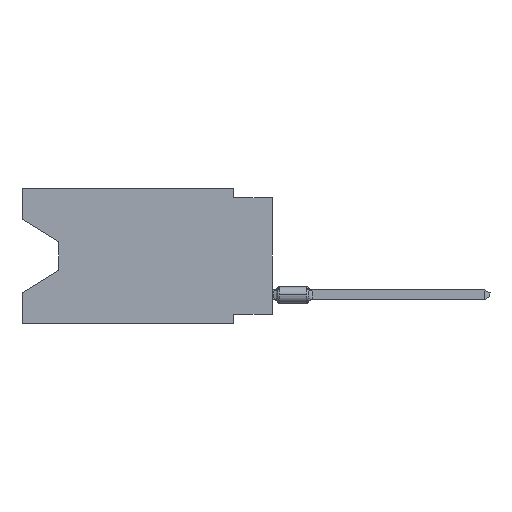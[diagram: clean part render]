
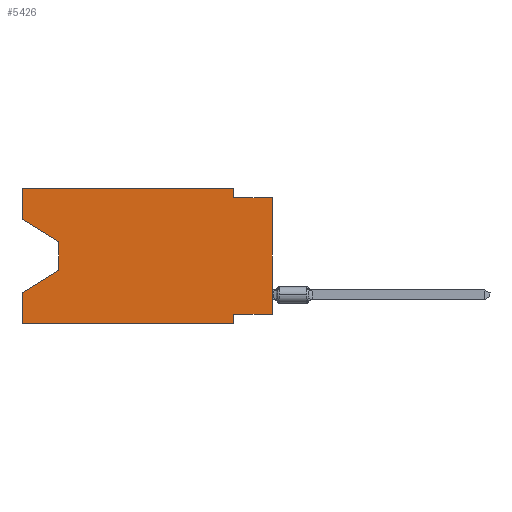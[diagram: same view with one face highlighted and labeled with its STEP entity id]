
A CAD part, left-side view. The second image highlights one B-rep face of the part: STEP entity #5426.
In plain terms, the highlighted planar face has unit normal (-1, 0, 0).
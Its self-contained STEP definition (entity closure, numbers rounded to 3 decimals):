
#700 = CARTESIAN_POINT ( 'NONE',  ( 0., 0., -0.635 ) ) ;
#1906 = EDGE_CURVE ( 'NONE', #69112, #50291, #23271, .T. ) ;
#2509 = CARTESIAN_POINT ( 'NONE',  ( 0., 2.54, 0. ) ) ;
#5221 = LINE ( 'NONE', #42777, #41281 ) ;
#5332 = CARTESIAN_POINT ( 'NONE',  ( 0., 16.383, 0. ) ) ;
#5359 = EDGE_CURVE ( 'NONE', #28296, #55410, #5221, .T. ) ;
#5382 = LINE ( 'NONE', #64990, #24940 ) ;
#5426 = ADVANCED_FACE ( 'NONE', ( #23437 ), #44844, .F. ) ;
#7646 = CARTESIAN_POINT ( 'NONE',  ( 0., 13.97, -3.505 ) ) ;
#7961 = LINE ( 'NONE', #40594, #66143 ) ;
#8326 = VECTOR ( 'NONE', #51748, 1000. ) ;
#8767 = LINE ( 'NONE', #30171, #30297 ) ;
#8883 = CARTESIAN_POINT ( 'NONE',  ( 0., 16.383, -6.852 ) ) ;
#8951 = LINE ( 'NONE', #68236, #39825 ) ;
#9491 = EDGE_CURVE ( 'NONE', #42059, #64264, #7961, .T. ) ;
#12438 = CARTESIAN_POINT ( 'NONE',  ( 0., 2.54, 0. ) ) ;
#12466 = EDGE_CURVE ( 'NONE', #66801, #26577, #39843, .T. ) ;
#12892 = CARTESIAN_POINT ( 'NONE',  ( 0., 13.97, -5.385 ) ) ;
#13167 = VERTEX_POINT ( 'NONE', #22146 ) ;
#13910 = DIRECTION ( 'NONE',  ( 0., -1., 0. ) ) ;
#16128 = VECTOR ( 'NONE', #19003, 1000. ) ;
#18149 = VECTOR ( 'NONE', #42419, 1000. ) ;
#18190 = VERTEX_POINT ( 'NONE', #53420 ) ;
#18641 = ORIENTED_EDGE ( 'NONE', *, *, #35057, .F. ) ;
#19003 = DIRECTION ( 'NONE',  ( 0., 0., -1. ) ) ;
#19448 = CARTESIAN_POINT ( 'NONE',  ( 0., 16.383, -2.038 ) ) ;
#21558 = EDGE_CURVE ( 'NONE', #66801, #59343, #8767, .T. ) ;
#22146 = CARTESIAN_POINT ( 'NONE',  ( 0., 0., -8.255 ) ) ;
#22384 = LINE ( 'NONE', #12892, #66435 ) ;
#23271 = LINE ( 'NONE', #54512, #66870 ) ;
#23437 = FACE_OUTER_BOUND ( 'NONE', #52277, .T. ) ;
#24940 = VECTOR ( 'NONE', #53801, 1000. ) ;
#25041 = EDGE_CURVE ( 'NONE', #18190, #26577, #5382, .T. ) ;
#25972 = EDGE_CURVE ( 'NONE', #50291, #59343, #22384, .T. ) ;
#26577 = VERTEX_POINT ( 'NONE', #58649 ) ;
#27580 = ORIENTED_EDGE ( 'NONE', *, *, #28864, .F. ) ;
#27849 = AXIS2_PLACEMENT_3D ( 'NONE', #34298, #56062, #49754 ) ;
#27957 = VECTOR ( 'NONE', #54413, 1000. ) ;
#28296 = VERTEX_POINT ( 'NONE', #19448 ) ;
#28528 = DIRECTION ( 'NONE',  ( 0., 1., 0. ) ) ;
#28864 = EDGE_CURVE ( 'NONE', #55410, #62103, #53718, .T. ) ;
#30171 = CARTESIAN_POINT ( 'NONE',  ( 0., 16.383, 0. ) ) ;
#30297 = VECTOR ( 'NONE', #51574, 1000. ) ;
#34298 = CARTESIAN_POINT ( 'NONE',  ( 0., 16.383, 0. ) ) ;
#35057 = EDGE_CURVE ( 'NONE', #62103, #42059, #35136, .T. ) ;
#35136 = LINE ( 'NONE', #2509, #16128 ) ;
#36466 = CARTESIAN_POINT ( 'NONE',  ( 0., 0., 0. ) ) ;
#39758 = DIRECTION ( 'NONE',  ( 0., 0., -1. ) ) ;
#39766 = CARTESIAN_POINT ( 'NONE',  ( 0., 13.97, -5.385 ) ) ;
#39825 = VECTOR ( 'NONE', #67891, 1000. ) ;
#39843 = LINE ( 'NONE', #55979, #8326 ) ;
#40594 = CARTESIAN_POINT ( 'NONE',  ( 0., 0., -0.635 ) ) ;
#40658 = VECTOR ( 'NONE', #28528, 1000. ) ;
#40787 = CARTESIAN_POINT ( 'NONE',  ( 0., 0., -8.255 ) ) ;
#41129 = ORIENTED_EDGE ( 'NONE', *, *, #52412, .T. ) ;
#41281 = VECTOR ( 'NONE', #69408, 1000. ) ;
#41924 = ORIENTED_EDGE ( 'NONE', *, *, #48989, .F. ) ;
#42059 = VERTEX_POINT ( 'NONE', #60523 ) ;
#42157 = CARTESIAN_POINT ( 'NONE',  ( 0., 16.383, 0. ) ) ;
#42419 = DIRECTION ( 'NONE',  ( 0., 0., 1. ) ) ;
#42777 = CARTESIAN_POINT ( 'NONE',  ( 0., 16.383, 0. ) ) ;
#44844 = PLANE ( 'NONE',  #27849 ) ;
#48580 = ORIENTED_EDGE ( 'NONE', *, *, #5359, .F. ) ;
#48989 = EDGE_CURVE ( 'NONE', #13167, #18190, #61831, .T. ) ;
#49754 = DIRECTION ( 'NONE',  ( 0., 0., -1. ) ) ;
#50291 = VERTEX_POINT ( 'NONE', #39766 ) ;
#50639 = ORIENTED_EDGE ( 'NONE', *, *, #25041, .F. ) ;
#51574 = DIRECTION ( 'NONE',  ( 0., 0., 1. ) ) ;
#51748 = DIRECTION ( 'NONE',  ( 0., -1., 0. ) ) ;
#52277 = EDGE_LOOP ( 'NONE', ( #41129, #58030, #65001, #65936, #62634, #50639, #41924, #61906, #67643, #18641, #27580, #48580 ) ) ;
#52412 = EDGE_CURVE ( 'NONE', #28296, #69112, #8951, .T. ) ;
#53420 = CARTESIAN_POINT ( 'NONE',  ( 0., 2.54, -8.255 ) ) ;
#53718 = LINE ( 'NONE', #42157, #27957 ) ;
#53801 = DIRECTION ( 'NONE',  ( 0., 0., -1. ) ) ;
#54333 = DIRECTION ( 'NONE',  ( 0., 0.855, -0.519 ) ) ;
#54413 = DIRECTION ( 'NONE',  ( 0., -1., 0. ) ) ;
#54512 = CARTESIAN_POINT ( 'NONE',  ( 0., 13.97, -3.505 ) ) ;
#55410 = VERTEX_POINT ( 'NONE', #5332 ) ;
#55979 = CARTESIAN_POINT ( 'NONE',  ( 0., 16.383, -8.89 ) ) ;
#56062 = DIRECTION ( 'NONE',  ( 1., 0., 0. ) ) ;
#58030 = ORIENTED_EDGE ( 'NONE', *, *, #1906, .T. ) ;
#58213 = LINE ( 'NONE', #36466, #18149 ) ;
#58649 = CARTESIAN_POINT ( 'NONE',  ( 0., 2.54, -8.89 ) ) ;
#59343 = VERTEX_POINT ( 'NONE', #8883 ) ;
#60523 = CARTESIAN_POINT ( 'NONE',  ( 0., 2.54, -0.635 ) ) ;
#61831 = LINE ( 'NONE', #40787, #40658 ) ;
#61906 = ORIENTED_EDGE ( 'NONE', *, *, #65932, .T. ) ;
#62103 = VERTEX_POINT ( 'NONE', #12438 ) ;
#62634 = ORIENTED_EDGE ( 'NONE', *, *, #12466, .T. ) ;
#62673 = CARTESIAN_POINT ( 'NONE',  ( 0., 16.383, -8.89 ) ) ;
#64264 = VERTEX_POINT ( 'NONE', #700 ) ;
#64990 = CARTESIAN_POINT ( 'NONE',  ( 0., 2.54, -8.89 ) ) ;
#65001 = ORIENTED_EDGE ( 'NONE', *, *, #25972, .T. ) ;
#65932 = EDGE_CURVE ( 'NONE', #13167, #64264, #58213, .T. ) ;
#65936 = ORIENTED_EDGE ( 'NONE', *, *, #21558, .F. ) ;
#66143 = VECTOR ( 'NONE', #13910, 1000. ) ;
#66435 = VECTOR ( 'NONE', #54333, 1000. ) ;
#66801 = VERTEX_POINT ( 'NONE', #62673 ) ;
#66870 = VECTOR ( 'NONE', #39758, 1000. ) ;
#67643 = ORIENTED_EDGE ( 'NONE', *, *, #9491, .F. ) ;
#67891 = DIRECTION ( 'NONE',  ( 0., -0.855, -0.519 ) ) ;
#68236 = CARTESIAN_POINT ( 'NONE',  ( 0., 16.383, -2.038 ) ) ;
#69112 = VERTEX_POINT ( 'NONE', #7646 ) ;
#69408 = DIRECTION ( 'NONE',  ( 0., 0., 1. ) ) ;
